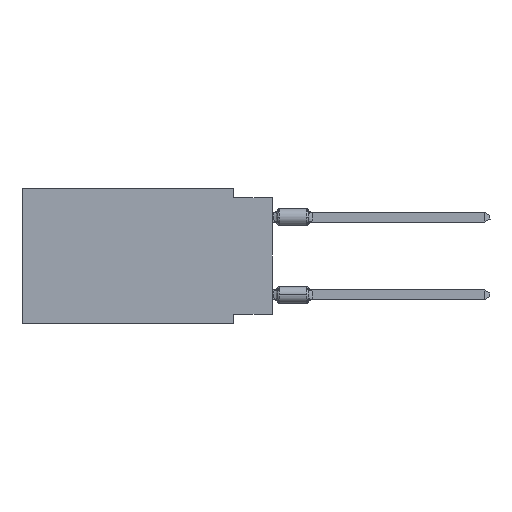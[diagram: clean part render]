
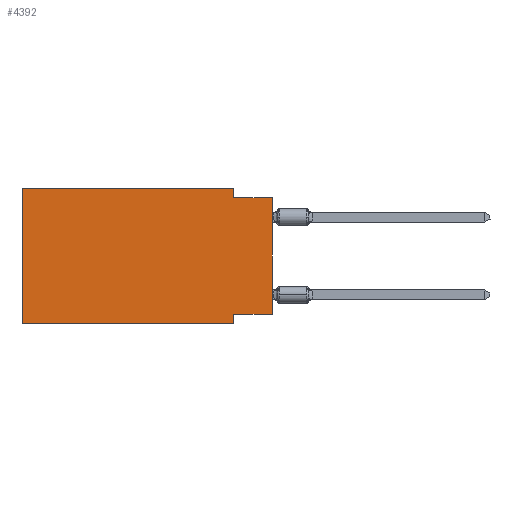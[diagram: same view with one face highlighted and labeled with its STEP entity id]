
A CAD part, left-side view. The second image highlights one B-rep face of the part: STEP entity #4392.
In plain terms, the highlighted planar face has unit normal (-1, 0, 0).
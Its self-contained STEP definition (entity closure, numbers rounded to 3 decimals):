
#795 = DIRECTION ( 'NONE',  ( 0., -1., 0. ) ) ;
#1969 = VERTEX_POINT ( 'NONE', #25167 ) ;
#2039 = EDGE_CURVE ( 'NONE', #13311, #10087, #19846, .T. ) ;
#2228 = EDGE_CURVE ( 'NONE', #2973, #14802, #11993, .T. ) ;
#2325 = DIRECTION ( 'NONE',  ( 0., 0., 1. ) ) ;
#2973 = VERTEX_POINT ( 'NONE', #11224 ) ;
#3510 = CARTESIAN_POINT ( 'NONE',  ( 0., 16.383, 0. ) ) ;
#3831 = CARTESIAN_POINT ( 'NONE',  ( 0., 16.383, -8.89 ) ) ;
#4215 = VECTOR ( 'NONE', #2325, 1000. ) ;
#4280 = VERTEX_POINT ( 'NONE', #17459 ) ;
#4392 = ADVANCED_FACE ( 'NONE', ( #30550 ), #17037, .F. ) ;
#6312 = DIRECTION ( 'NONE',  ( 0., -1., 0. ) ) ;
#6802 = EDGE_CURVE ( 'NONE', #14802, #7638, #31459, .T. ) ;
#7638 = VERTEX_POINT ( 'NONE', #11016 ) ;
#8124 = LINE ( 'NONE', #15984, #27083 ) ;
#8457 = LINE ( 'NONE', #19305, #17668 ) ;
#9527 = DIRECTION ( 'NONE',  ( 0., 1., 0. ) ) ;
#9761 = EDGE_CURVE ( 'NONE', #19455, #7638, #19839, .T. ) ;
#10087 = VERTEX_POINT ( 'NONE', #26756 ) ;
#10492 = LINE ( 'NONE', #26175, #4215 ) ;
#11016 = CARTESIAN_POINT ( 'NONE',  ( 0., 2.54, -8.89 ) ) ;
#11224 = CARTESIAN_POINT ( 'NONE',  ( 0., 0., -8.255 ) ) ;
#11628 = VECTOR ( 'NONE', #9527, 1000. ) ;
#11680 = DIRECTION ( 'NONE',  ( 0., 0., -1. ) ) ;
#11993 = LINE ( 'NONE', #28379, #11628 ) ;
#12906 = AXIS2_PLACEMENT_3D ( 'NONE', #3510, #25203, #11680 ) ;
#13311 = VERTEX_POINT ( 'NONE', #33077 ) ;
#13335 = VECTOR ( 'NONE', #795, 1000. ) ;
#13722 = EDGE_CURVE ( 'NONE', #1969, #4280, #8457, .T. ) ;
#14802 = VERTEX_POINT ( 'NONE', #29665 ) ;
#15237 = EDGE_CURVE ( 'NONE', #4280, #13311, #21468, .T. ) ;
#15984 = CARTESIAN_POINT ( 'NONE',  ( 0., 0., 0. ) ) ;
#16470 = CARTESIAN_POINT ( 'NONE',  ( 0., 2.54, 0. ) ) ;
#16935 = ORIENTED_EDGE ( 'NONE', *, *, #15237, .F. ) ;
#17037 = PLANE ( 'NONE',  #12906 ) ;
#17459 = CARTESIAN_POINT ( 'NONE',  ( 0., 2.54, 0. ) ) ;
#17668 = VECTOR ( 'NONE', #30138, 1000. ) ;
#18153 = CARTESIAN_POINT ( 'NONE',  ( 0., 2.54, -8.89 ) ) ;
#19305 = CARTESIAN_POINT ( 'NONE',  ( 0., 16.383, 0. ) ) ;
#19455 = VERTEX_POINT ( 'NONE', #21791 ) ;
#19839 = LINE ( 'NONE', #3831, #13335 ) ;
#19846 = LINE ( 'NONE', #30680, #28118 ) ;
#21413 = VECTOR ( 'NONE', #27307, 1000. ) ;
#21468 = LINE ( 'NONE', #16470, #21413 ) ;
#21656 = DIRECTION ( 'NONE',  ( 0., 0., 1. ) ) ;
#21791 = CARTESIAN_POINT ( 'NONE',  ( 0., 16.383, -8.89 ) ) ;
#23276 = ORIENTED_EDGE ( 'NONE', *, *, #2039, .F. ) ;
#23635 = VECTOR ( 'NONE', #28977, 1000. ) ;
#23992 = EDGE_CURVE ( 'NONE', #19455, #1969, #10492, .T. ) ;
#25167 = CARTESIAN_POINT ( 'NONE',  ( 0., 16.383, 0. ) ) ;
#25203 = DIRECTION ( 'NONE',  ( 1., 0., 0. ) ) ;
#25518 = ORIENTED_EDGE ( 'NONE', *, *, #13722, .F. ) ;
#26175 = CARTESIAN_POINT ( 'NONE',  ( 0., 16.383, 0. ) ) ;
#26756 = CARTESIAN_POINT ( 'NONE',  ( 0., 0., -0.635 ) ) ;
#27083 = VECTOR ( 'NONE', #21656, 1000. ) ;
#27307 = DIRECTION ( 'NONE',  ( 0., 0., -1. ) ) ;
#28118 = VECTOR ( 'NONE', #6312, 1000. ) ;
#28379 = CARTESIAN_POINT ( 'NONE',  ( 0., 0., -8.255 ) ) ;
#28977 = DIRECTION ( 'NONE',  ( 0., 0., -1. ) ) ;
#29153 = ORIENTED_EDGE ( 'NONE', *, *, #23992, .F. ) ;
#29344 = ORIENTED_EDGE ( 'NONE', *, *, #2228, .F. ) ;
#29665 = CARTESIAN_POINT ( 'NONE',  ( 0., 2.54, -8.255 ) ) ;
#30138 = DIRECTION ( 'NONE',  ( 0., -1., 0. ) ) ;
#30550 = FACE_OUTER_BOUND ( 'NONE', #31534, .T. ) ;
#30680 = CARTESIAN_POINT ( 'NONE',  ( 0., 0., -0.635 ) ) ;
#31459 = LINE ( 'NONE', #18153, #23635 ) ;
#31534 = EDGE_LOOP ( 'NONE', ( #33609, #23276, #16935, #25518, #29153, #34899, #31969, #29344 ) ) ;
#31969 = ORIENTED_EDGE ( 'NONE', *, *, #6802, .F. ) ;
#33077 = CARTESIAN_POINT ( 'NONE',  ( 0., 2.54, -0.635 ) ) ;
#33609 = ORIENTED_EDGE ( 'NONE', *, *, #34760, .T. ) ;
#34760 = EDGE_CURVE ( 'NONE', #2973, #10087, #8124, .T. ) ;
#34899 = ORIENTED_EDGE ( 'NONE', *, *, #9761, .T. ) ;
